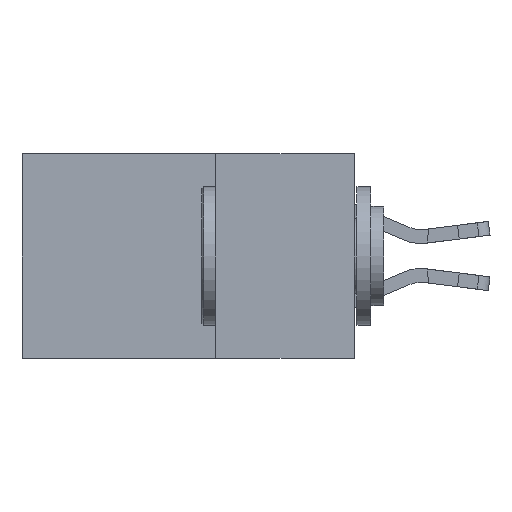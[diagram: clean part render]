
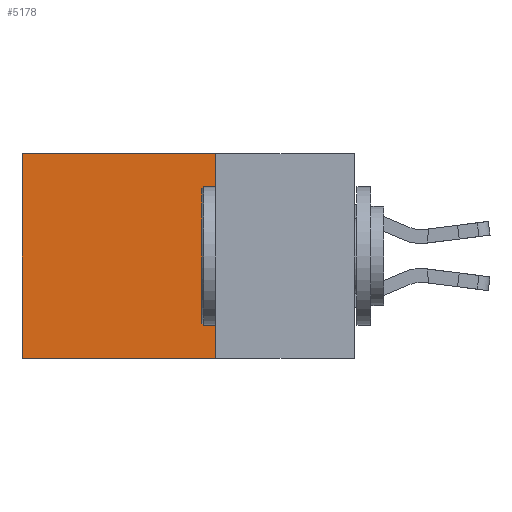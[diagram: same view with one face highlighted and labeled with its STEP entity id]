
A CAD part, left-side view. The second image highlights one B-rep face of the part: STEP entity #5178.
In plain terms, the highlighted planar face has unit normal (-1, 0, 0).
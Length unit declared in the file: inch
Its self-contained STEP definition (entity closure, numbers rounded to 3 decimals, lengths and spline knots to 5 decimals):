
#577 = CARTESIAN_POINT ( 'NONE',  ( 0.2615, 0.25, -0.37 ) ) ;
#1098 = VECTOR ( 'NONE', #3476, 39.37008 ) ;
#1207 = ORIENTED_EDGE ( 'NONE', *, *, #10232, .T. ) ;
#1407 = VERTEX_POINT ( 'NONE', #577 ) ;
#2632 = CARTESIAN_POINT ( 'NONE',  ( 0.2615, 0.25, 0. ) ) ;
#2974 = CARTESIAN_POINT ( 'NONE',  ( 0.2615, 0.6, -0.37 ) ) ;
#3324 = LINE ( 'NONE', #20750, #21823 ) ;
#3476 = DIRECTION ( 'NONE',  ( 0., 0., -1. ) ) ;
#4380 = FACE_OUTER_BOUND ( 'NONE', #4449, .T. ) ;
#4449 = EDGE_LOOP ( 'NONE', ( #1207, #19275, #11438, #9979 ) ) ;
#4875 = VECTOR ( 'NONE', #8086, 39.37008 ) ;
#5178 = ADVANCED_FACE ( 'NONE', ( #4380 ), #14712, .F. ) ;
#6011 = LINE ( 'NONE', #23132, #1098 ) ;
#8086 = DIRECTION ( 'NONE',  ( 0., 1., 0. ) ) ;
#8161 = VERTEX_POINT ( 'NONE', #2974 ) ;
#8614 = AXIS2_PLACEMENT_3D ( 'NONE', #14431, #14410, #14342 ) ;
#9979 = ORIENTED_EDGE ( 'NONE', *, *, #22153, .T. ) ;
#10195 = CARTESIAN_POINT ( 'NONE',  ( 0.2615, 0.25, -0.37 ) ) ;
#10232 = EDGE_CURVE ( 'NONE', #16086, #8161, #6011, .T. ) ;
#11277 = LINE ( 'NONE', #2632, #4875 ) ;
#11395 = VECTOR ( 'NONE', #12021, 39.37008 ) ;
#11438 = ORIENTED_EDGE ( 'NONE', *, *, #15104, .F. ) ;
#11787 = DIRECTION ( 'NONE',  ( 0., 0., -1. ) ) ;
#12021 = DIRECTION ( 'NONE',  ( 0., 1., 0. ) ) ;
#12175 = VERTEX_POINT ( 'NONE', #15721 ) ;
#14342 = DIRECTION ( 'NONE',  ( 0., 0., -1. ) ) ;
#14410 = DIRECTION ( 'NONE',  ( 1., 0., 0. ) ) ;
#14431 = CARTESIAN_POINT ( 'NONE',  ( 0.2615, 0.25, -0.37 ) ) ;
#14712 = PLANE ( 'NONE',  #8614 ) ;
#15104 = EDGE_CURVE ( 'NONE', #12175, #1407, #3324, .T. ) ;
#15721 = CARTESIAN_POINT ( 'NONE',  ( 0.2615, 0.25, 0. ) ) ;
#16086 = VERTEX_POINT ( 'NONE', #17397 ) ;
#17331 = LINE ( 'NONE', #10195, #11395 ) ;
#17397 = CARTESIAN_POINT ( 'NONE',  ( 0.2615, 0.6, 0. ) ) ;
#19275 = ORIENTED_EDGE ( 'NONE', *, *, #19785, .F. ) ;
#19785 = EDGE_CURVE ( 'NONE', #1407, #8161, #17331, .T. ) ;
#20750 = CARTESIAN_POINT ( 'NONE',  ( 0.2615, 0.25, -0.37 ) ) ;
#21823 = VECTOR ( 'NONE', #11787, 39.37008 ) ;
#22153 = EDGE_CURVE ( 'NONE', #12175, #16086, #11277, .T. ) ;
#23132 = CARTESIAN_POINT ( 'NONE',  ( 0.2615, 0.6, -0.37 ) ) ;
